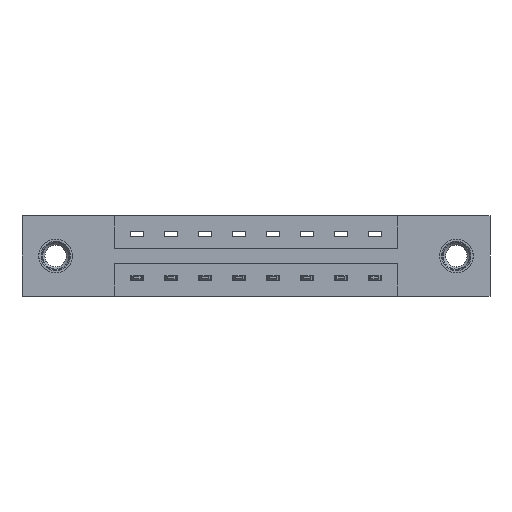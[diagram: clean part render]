
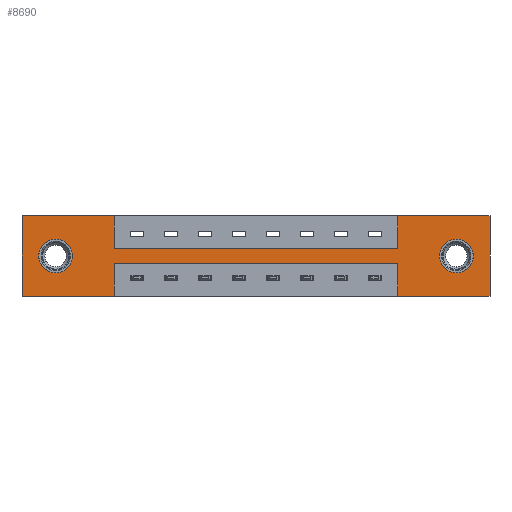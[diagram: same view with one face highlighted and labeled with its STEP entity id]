
A CAD part, front view. The second image highlights one B-rep face of the part: STEP entity #8690.
In plain terms, the highlighted planar face has unit normal (0, -1, 0).
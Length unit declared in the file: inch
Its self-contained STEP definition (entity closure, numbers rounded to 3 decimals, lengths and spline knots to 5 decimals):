
#172 = ORIENTED_EDGE ( 'NONE', *, *, #4939, .T. ) ;
#246 = AXIS2_PLACEMENT_3D ( 'NONE', #6757, #10283, #11267 ) ;
#249 = EDGE_CURVE ( 'NONE', #9367, #3299, #3019, .T. ) ;
#417 = VECTOR ( 'NONE', #9521, 39.37008 ) ;
#538 = VECTOR ( 'NONE', #9213, 39.37008 ) ;
#561 = CARTESIAN_POINT ( 'NONE',  ( 1.729, 0., -0.37 ) ) ;
#599 = CARTESIAN_POINT ( 'NONE',  ( 1.729, 0., -0.22 ) ) ;
#607 = CARTESIAN_POINT ( 'NONE',  ( 1.999, 0., -0.185 ) ) ;
#713 = DIRECTION ( 'NONE',  ( 0., 0., -1. ) ) ;
#834 = FACE_OUTER_BOUND ( 'NONE', #3914, .T. ) ;
#931 = CARTESIAN_POINT ( 'NONE',  ( 1.729, 0., 0. ) ) ;
#957 = CARTESIAN_POINT ( 'NONE',  ( 0.425, 0., -0.37 ) ) ;
#1078 = DIRECTION ( 'NONE',  ( 1., 0., 0. ) ) ;
#1138 = AXIS2_PLACEMENT_3D ( 'NONE', #1454, #4877, #2294 ) ;
#1367 = FACE_BOUND ( 'NONE', #8385, .T. ) ;
#1447 = EDGE_CURVE ( 'NONE', #9911, #7333, #9870, .T. ) ;
#1454 = CARTESIAN_POINT ( 'NONE',  ( 1.999, 0., -0.185 ) ) ;
#1512 = EDGE_CURVE ( 'NONE', #5629, #5912, #5568, .T. ) ;
#1657 = ORIENTED_EDGE ( 'NONE', *, *, #9240, .F. ) ;
#1883 = LINE ( 'NONE', #7827, #4489 ) ;
#1893 = AXIS2_PLACEMENT_3D ( 'NONE', #6525, #7438, #5673 ) ;
#2012 = CIRCLE ( 'NONE', #1893, 0.078 ) ;
#2034 = LINE ( 'NONE', #9359, #9748 ) ;
#2117 = CARTESIAN_POINT ( 'NONE',  ( 1.999, 0., -0.107 ) ) ;
#2138 = EDGE_CURVE ( 'NONE', #5779, #9668, #2277, .T. ) ;
#2214 = CARTESIAN_POINT ( 'NONE',  ( 0.155, 0., -0.263 ) ) ;
#2277 = CIRCLE ( 'NONE', #1138, 0.078 ) ;
#2294 = DIRECTION ( 'NONE',  ( 0., 0., -1. ) ) ;
#2442 = DIRECTION ( 'NONE',  ( 1., 0., 0. ) ) ;
#2752 = CARTESIAN_POINT ( 'NONE',  ( 0.425, 0., -0.22 ) ) ;
#3019 = LINE ( 'NONE', #3887, #9900 ) ;
#3066 = ORIENTED_EDGE ( 'NONE', *, *, #10689, .T. ) ;
#3158 = VERTEX_POINT ( 'NONE', #2214 ) ;
#3232 = ORIENTED_EDGE ( 'NONE', *, *, #2138, .T. ) ;
#3269 = VECTOR ( 'NONE', #5463, 39.37008 ) ;
#3299 = VERTEX_POINT ( 'NONE', #5483 ) ;
#3334 = LINE ( 'NONE', #8680, #11046 ) ;
#3553 = EDGE_CURVE ( 'NONE', #6444, #9383, #3689, .T. ) ;
#3650 = ORIENTED_EDGE ( 'NONE', *, *, #8720, .F. ) ;
#3689 = LINE ( 'NONE', #5284, #4235 ) ;
#3852 = CARTESIAN_POINT ( 'NONE',  ( 0.425, 0., 0. ) ) ;
#3853 = EDGE_CURVE ( 'NONE', #3299, #8351, #10846, .T. ) ;
#3886 = EDGE_CURVE ( 'NONE', #3988, #6444, #2034, .T. ) ;
#3887 = CARTESIAN_POINT ( 'NONE',  ( 0., 0., 0. ) ) ;
#3914 = EDGE_LOOP ( 'NONE', ( #5112, #6455, #1657, #7294, #9698, #6579, #10884, #3650, #10518, #9674, #5299, #6321 ) ) ;
#3988 = VERTEX_POINT ( 'NONE', #7851 ) ;
#3994 = DIRECTION ( 'NONE',  ( 0., 0., 1. ) ) ;
#4065 = CIRCLE ( 'NONE', #5909, 0.078 ) ;
#4235 = VECTOR ( 'NONE', #1078, 39.37008 ) ;
#4261 = LINE ( 'NONE', #9500, #5738 ) ;
#4267 = EDGE_LOOP ( 'NONE', ( #172, #3066 ) ) ;
#4419 = DIRECTION ( 'NONE',  ( 0., 0., 1. ) ) ;
#4489 = VECTOR ( 'NONE', #4531, 39.37008 ) ;
#4531 = DIRECTION ( 'NONE',  ( -1., 0., 0. ) ) ;
#4877 = DIRECTION ( 'NONE',  ( 0., 1., 0. ) ) ;
#4939 = EDGE_CURVE ( 'NONE', #9969, #3158, #2012, .T. ) ;
#4957 = DIRECTION ( 'NONE',  ( 0., 0., 1. ) ) ;
#5112 = ORIENTED_EDGE ( 'NONE', *, *, #9390, .F. ) ;
#5196 = VECTOR ( 'NONE', #3994, 39.37008 ) ;
#5284 = CARTESIAN_POINT ( 'NONE',  ( 0., 0., 0. ) ) ;
#5299 = ORIENTED_EDGE ( 'NONE', *, *, #7304, .F. ) ;
#5378 = LINE ( 'NONE', #6894, #7995 ) ;
#5421 = CIRCLE ( 'NONE', #10406, 0.078 ) ;
#5463 = DIRECTION ( 'NONE',  ( -1., 0., 0. ) ) ;
#5483 = CARTESIAN_POINT ( 'NONE',  ( 0.425, 0., 0. ) ) ;
#5495 = CARTESIAN_POINT ( 'NONE',  ( 0.155, 0., -0.107 ) ) ;
#5568 = LINE ( 'NONE', #9919, #3269 ) ;
#5574 = DIRECTION ( 'NONE',  ( -1., 0., 0. ) ) ;
#5629 = VERTEX_POINT ( 'NONE', #7667 ) ;
#5670 = EDGE_CURVE ( 'NONE', #9668, #5779, #4065, .T. ) ;
#5673 = DIRECTION ( 'NONE',  ( 0., 0., 1. ) ) ;
#5738 = VECTOR ( 'NONE', #2442, 39.37008 ) ;
#5779 = VERTEX_POINT ( 'NONE', #2117 ) ;
#5819 = VERTEX_POINT ( 'NONE', #957 ) ;
#5909 = AXIS2_PLACEMENT_3D ( 'NONE', #607, #6734, #713 ) ;
#5912 = VERTEX_POINT ( 'NONE', #561 ) ;
#6126 = VECTOR ( 'NONE', #5574, 39.37008 ) ;
#6321 = ORIENTED_EDGE ( 'NONE', *, *, #10950, .F. ) ;
#6444 = VERTEX_POINT ( 'NONE', #931 ) ;
#6455 = ORIENTED_EDGE ( 'NONE', *, *, #1447, .F. ) ;
#6525 = CARTESIAN_POINT ( 'NONE',  ( 0.155, 0., -0.185 ) ) ;
#6536 = CARTESIAN_POINT ( 'NONE',  ( 1.729, 0., -0.37 ) ) ;
#6579 = ORIENTED_EDGE ( 'NONE', *, *, #3553, .F. ) ;
#6734 = DIRECTION ( 'NONE',  ( 0., 1., 0. ) ) ;
#6757 = CARTESIAN_POINT ( 'NONE',  ( 0., 0., -0.37 ) ) ;
#6758 = ORIENTED_EDGE ( 'NONE', *, *, #5670, .T. ) ;
#6803 = DIRECTION ( 'NONE',  ( 0., 0., 1. ) ) ;
#6894 = CARTESIAN_POINT ( 'NONE',  ( 2.154, 0., 0. ) ) ;
#7122 = CARTESIAN_POINT ( 'NONE',  ( 0.425, 0., -0.15 ) ) ;
#7294 = ORIENTED_EDGE ( 'NONE', *, *, #1512, .F. ) ;
#7302 = EDGE_CURVE ( 'NONE', #9383, #5629, #5378, .T. ) ;
#7304 = EDGE_CURVE ( 'NONE', #8123, #9367, #3334, .T. ) ;
#7333 = VERTEX_POINT ( 'NONE', #8449 ) ;
#7438 = DIRECTION ( 'NONE',  ( 0., 1., 0. ) ) ;
#7496 = CARTESIAN_POINT ( 'NONE',  ( 0., 0., -0.37 ) ) ;
#7667 = CARTESIAN_POINT ( 'NONE',  ( 2.154, 0., -0.37 ) ) ;
#7827 = CARTESIAN_POINT ( 'NONE',  ( 0., 0., -0.37 ) ) ;
#7851 = CARTESIAN_POINT ( 'NONE',  ( 1.729, 0., -0.15 ) ) ;
#7995 = VECTOR ( 'NONE', #9702, 39.37008 ) ;
#8123 = VERTEX_POINT ( 'NONE', #7496 ) ;
#8124 = CARTESIAN_POINT ( 'NONE',  ( 1.999, 0., -0.263 ) ) ;
#8351 = VERTEX_POINT ( 'NONE', #7122 ) ;
#8376 = CARTESIAN_POINT ( 'NONE',  ( 0.155, 0., -0.185 ) ) ;
#8385 = EDGE_LOOP ( 'NONE', ( #3232, #6758 ) ) ;
#8449 = CARTESIAN_POINT ( 'NONE',  ( 0.425, 0., -0.22 ) ) ;
#8592 = CARTESIAN_POINT ( 'NONE',  ( 0.425, 0., -0.37 ) ) ;
#8643 = LINE ( 'NONE', #6536, #5196 ) ;
#8680 = CARTESIAN_POINT ( 'NONE',  ( 0., 0., 0. ) ) ;
#8690 = ADVANCED_FACE ( 'NONE', ( #1367, #10452, #834 ), #11201, .T. ) ;
#8720 = EDGE_CURVE ( 'NONE', #8351, #3988, #4261, .T. ) ;
#9213 = DIRECTION ( 'NONE',  ( 0., 0., -1. ) ) ;
#9240 = EDGE_CURVE ( 'NONE', #5912, #9911, #8643, .T. ) ;
#9359 = CARTESIAN_POINT ( 'NONE',  ( 1.729, 0., 0. ) ) ;
#9367 = VERTEX_POINT ( 'NONE', #10862 ) ;
#9383 = VERTEX_POINT ( 'NONE', #10058 ) ;
#9390 = EDGE_CURVE ( 'NONE', #7333, #5819, #10298, .T. ) ;
#9500 = CARTESIAN_POINT ( 'NONE',  ( 0.425, 0., -0.15 ) ) ;
#9521 = DIRECTION ( 'NONE',  ( 0., 0., -1. ) ) ;
#9668 = VERTEX_POINT ( 'NONE', #8124 ) ;
#9674 = ORIENTED_EDGE ( 'NONE', *, *, #249, .F. ) ;
#9698 = ORIENTED_EDGE ( 'NONE', *, *, #7302, .F. ) ;
#9702 = DIRECTION ( 'NONE',  ( 0., 0., -1. ) ) ;
#9748 = VECTOR ( 'NONE', #6803, 39.37008 ) ;
#9870 = LINE ( 'NONE', #2752, #6126 ) ;
#9900 = VECTOR ( 'NONE', #10921, 39.37008 ) ;
#9911 = VERTEX_POINT ( 'NONE', #599 ) ;
#9919 = CARTESIAN_POINT ( 'NONE',  ( 0., 0., -0.37 ) ) ;
#9969 = VERTEX_POINT ( 'NONE', #5495 ) ;
#10058 = CARTESIAN_POINT ( 'NONE',  ( 2.154, 0., 0. ) ) ;
#10195 = DIRECTION ( 'NONE',  ( 0., 1., 0. ) ) ;
#10283 = DIRECTION ( 'NONE',  ( 0., -1., 0. ) ) ;
#10298 = LINE ( 'NONE', #8592, #417 ) ;
#10406 = AXIS2_PLACEMENT_3D ( 'NONE', #8376, #10195, #4957 ) ;
#10452 = FACE_BOUND ( 'NONE', #4267, .T. ) ;
#10518 = ORIENTED_EDGE ( 'NONE', *, *, #3853, .F. ) ;
#10689 = EDGE_CURVE ( 'NONE', #3158, #9969, #5421, .T. ) ;
#10846 = LINE ( 'NONE', #3852, #538 ) ;
#10862 = CARTESIAN_POINT ( 'NONE',  ( 0., 0., 0. ) ) ;
#10884 = ORIENTED_EDGE ( 'NONE', *, *, #3886, .F. ) ;
#10921 = DIRECTION ( 'NONE',  ( 1., 0., 0. ) ) ;
#10950 = EDGE_CURVE ( 'NONE', #5819, #8123, #1883, .T. ) ;
#11046 = VECTOR ( 'NONE', #4419, 39.37008 ) ;
#11201 = PLANE ( 'NONE',  #246 ) ;
#11267 = DIRECTION ( 'NONE',  ( 0., 0., -1. ) ) ;
